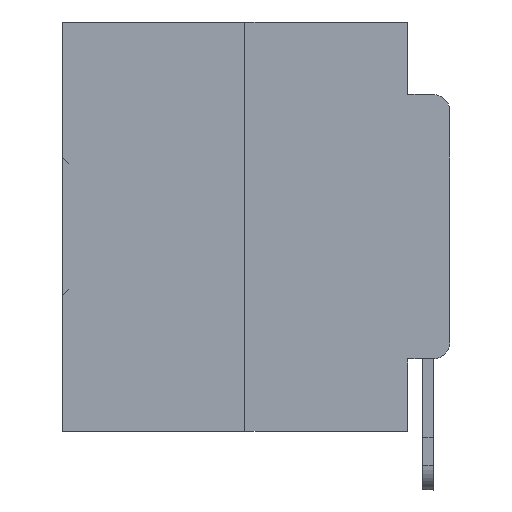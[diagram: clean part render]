
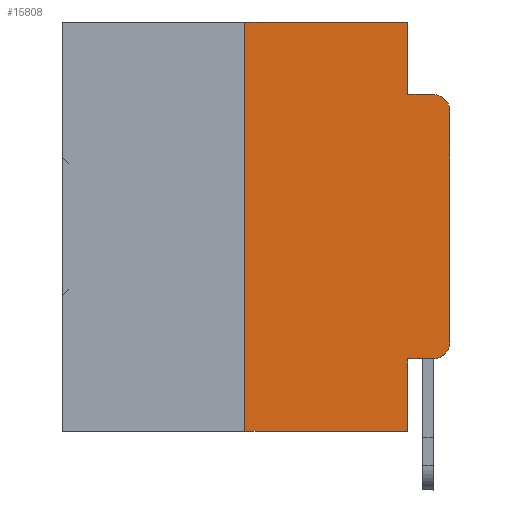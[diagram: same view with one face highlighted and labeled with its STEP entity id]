
A CAD part, left-side view. The second image highlights one B-rep face of the part: STEP entity #15808.
In plain terms, the highlighted planar face has unit normal (-1, 0, 0).
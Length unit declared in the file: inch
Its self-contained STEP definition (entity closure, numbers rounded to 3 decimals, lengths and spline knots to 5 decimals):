
#1201 = VERTEX_POINT ( 'NONE', #3443 ) ;
#1506 = DIRECTION ( 'NONE',  ( -1., 0., 0. ) ) ;
#2712 = CARTESIAN_POINT ( 'NONE',  ( 0., 0.02, -0.4115 ) ) ;
#3386 = EDGE_CURVE ( 'NONE', #31810, #1201, #10883, .T. ) ;
#3443 = CARTESIAN_POINT ( 'NONE',  ( 0., 0.02, -0.0885 ) ) ;
#3538 = VECTOR ( 'NONE', #24020, 39.37008 ) ;
#4122 = LINE ( 'NONE', #10124, #7906 ) ;
#4260 = CARTESIAN_POINT ( 'NONE',  ( 0., 0.25, -0.5 ) ) ;
#4348 = CARTESIAN_POINT ( 'NONE',  ( 0., 0., 0. ) ) ;
#4917 = ORIENTED_EDGE ( 'NONE', *, *, #34590, .T. ) ;
#5218 = CARTESIAN_POINT ( 'NONE',  ( 0., 0.051, -0.4115 ) ) ;
#5442 = VECTOR ( 'NONE', #29838, 39.37008 ) ;
#5623 = LINE ( 'NONE', #9648, #33294 ) ;
#5784 = CARTESIAN_POINT ( 'NONE',  ( 0., 0.473, 0. ) ) ;
#5841 = EDGE_CURVE ( 'NONE', #31910, #1201, #20489, .T. ) ;
#5893 = CARTESIAN_POINT ( 'NONE',  ( 0., 0.051, 0. ) ) ;
#5906 = VECTOR ( 'NONE', #19022, 39.37008 ) ;
#7215 = CIRCLE ( 'NONE', #11243, 0.02 ) ;
#7490 = CARTESIAN_POINT ( 'NONE',  ( 0., 0.02, -0.1085 ) ) ;
#7906 = VECTOR ( 'NONE', #15440, 39.37008 ) ;
#9642 = VECTOR ( 'NONE', #31447, 39.37008 ) ;
#9648 = CARTESIAN_POINT ( 'NONE',  ( 0., 0.25, 0. ) ) ;
#10117 = VERTEX_POINT ( 'NONE', #25099 ) ;
#10124 = CARTESIAN_POINT ( 'NONE',  ( 0., 0.051, 0. ) ) ;
#10687 = LINE ( 'NONE', #5218, #3538 ) ;
#10883 = CIRCLE ( 'NONE', #31831, 0.02 ) ;
#11243 = AXIS2_PLACEMENT_3D ( 'NONE', #17640, #1506, #20363 ) ;
#11262 = EDGE_CURVE ( 'NONE', #32462, #31910, #4122, .T. ) ;
#11295 = ORIENTED_EDGE ( 'NONE', *, *, #3386, .T. ) ;
#11307 = DIRECTION ( 'NONE',  ( 0., -1., 0. ) ) ;
#12054 = LINE ( 'NONE', #19873, #21390 ) ;
#12121 = LINE ( 'NONE', #5784, #5442 ) ;
#12692 = LINE ( 'NONE', #5893, #5906 ) ;
#13623 = CARTESIAN_POINT ( 'NONE',  ( 0., 0.051, -0.0885 ) ) ;
#14326 = ORIENTED_EDGE ( 'NONE', *, *, #26106, .T. ) ;
#15440 = DIRECTION ( 'NONE',  ( 0., 0., -1. ) ) ;
#15709 = EDGE_CURVE ( 'NONE', #34208, #21240, #7215, .T. ) ;
#15808 = ADVANCED_FACE ( 'NONE', ( #33185 ), #31200, .F. ) ;
#16720 = EDGE_CURVE ( 'NONE', #10117, #32462, #12121, .T. ) ;
#16929 = ORIENTED_EDGE ( 'NONE', *, *, #15709, .T. ) ;
#17640 = CARTESIAN_POINT ( 'NONE',  ( 0., 0.02, -0.3915 ) ) ;
#17799 = DIRECTION ( 'NONE',  ( 0., 0., 1. ) ) ;
#18068 = EDGE_CURVE ( 'NONE', #23235, #28985, #12054, .T. ) ;
#18123 = DIRECTION ( 'NONE',  ( 0., 0., -1. ) ) ;
#18348 = ORIENTED_EDGE ( 'NONE', *, *, #32202, .F. ) ;
#18632 = CARTESIAN_POINT ( 'NONE',  ( 0., 0., -0.3915 ) ) ;
#18872 = CARTESIAN_POINT ( 'NONE',  ( 0., 0.051, 0. ) ) ;
#19022 = DIRECTION ( 'NONE',  ( 0., 0., -1. ) ) ;
#19873 = CARTESIAN_POINT ( 'NONE',  ( 0., 0.473, -0.5 ) ) ;
#20363 = DIRECTION ( 'NONE',  ( 0., 0., -1. ) ) ;
#20489 = LINE ( 'NONE', #13623, #23385 ) ;
#20829 = DIRECTION ( 'NONE',  ( -1., 0., 0. ) ) ;
#21068 = CARTESIAN_POINT ( 'NONE',  ( 0., 0.051, -0.4115 ) ) ;
#21240 = VERTEX_POINT ( 'NONE', #18632 ) ;
#21364 = EDGE_LOOP ( 'NONE', ( #4917, #11295, #23291, #21726, #32823, #18348, #27681, #26021, #14326, #16929 ) ) ;
#21390 = VECTOR ( 'NONE', #11307, 39.37008 ) ;
#21495 = LINE ( 'NONE', #4348, #9642 ) ;
#21726 = ORIENTED_EDGE ( 'NONE', *, *, #11262, .F. ) ;
#23235 = VERTEX_POINT ( 'NONE', #4260 ) ;
#23291 = ORIENTED_EDGE ( 'NONE', *, *, #5841, .F. ) ;
#23385 = VECTOR ( 'NONE', #34741, 39.37008 ) ;
#24020 = DIRECTION ( 'NONE',  ( 0., -1., 0. ) ) ;
#24036 = CARTESIAN_POINT ( 'NONE',  ( 0., 0.051, -0.0885 ) ) ;
#25099 = CARTESIAN_POINT ( 'NONE',  ( 0., 0.25, 0. ) ) ;
#26021 = ORIENTED_EDGE ( 'NONE', *, *, #33526, .F. ) ;
#26106 = EDGE_CURVE ( 'NONE', #29375, #34208, #10687, .T. ) ;
#26143 = CARTESIAN_POINT ( 'NONE',  ( 0., 0.473, 0. ) ) ;
#27681 = ORIENTED_EDGE ( 'NONE', *, *, #18068, .T. ) ;
#28598 = AXIS2_PLACEMENT_3D ( 'NONE', #26143, #33900, #18123 ) ;
#28701 = CARTESIAN_POINT ( 'NONE',  ( 0., 0., -0.1085 ) ) ;
#28985 = VERTEX_POINT ( 'NONE', #30240 ) ;
#29375 = VERTEX_POINT ( 'NONE', #21068 ) ;
#29838 = DIRECTION ( 'NONE',  ( 0., -1., 0. ) ) ;
#30240 = CARTESIAN_POINT ( 'NONE',  ( 0., 0.051, -0.5 ) ) ;
#31200 = PLANE ( 'NONE',  #28598 ) ;
#31447 = DIRECTION ( 'NONE',  ( 0., 0., 1. ) ) ;
#31772 = DIRECTION ( 'NONE',  ( 0., 0., -1. ) ) ;
#31810 = VERTEX_POINT ( 'NONE', #28701 ) ;
#31831 = AXIS2_PLACEMENT_3D ( 'NONE', #7490, #20829, #31772 ) ;
#31910 = VERTEX_POINT ( 'NONE', #24036 ) ;
#32202 = EDGE_CURVE ( 'NONE', #23235, #10117, #5623, .T. ) ;
#32462 = VERTEX_POINT ( 'NONE', #18872 ) ;
#32823 = ORIENTED_EDGE ( 'NONE', *, *, #16720, .F. ) ;
#33185 = FACE_OUTER_BOUND ( 'NONE', #21364, .T. ) ;
#33294 = VECTOR ( 'NONE', #17799, 39.37008 ) ;
#33526 = EDGE_CURVE ( 'NONE', #29375, #28985, #12692, .T. ) ;
#33900 = DIRECTION ( 'NONE',  ( 1., 0., 0. ) ) ;
#34208 = VERTEX_POINT ( 'NONE', #2712 ) ;
#34590 = EDGE_CURVE ( 'NONE', #21240, #31810, #21495, .T. ) ;
#34741 = DIRECTION ( 'NONE',  ( 0., -1., 0. ) ) ;
